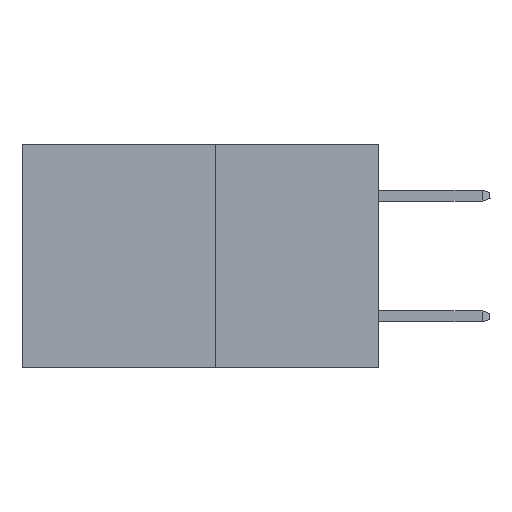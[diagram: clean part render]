
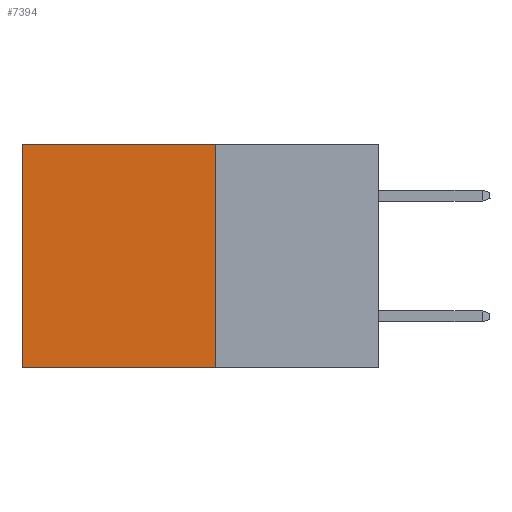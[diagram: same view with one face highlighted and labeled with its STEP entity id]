
A CAD part, left-side view. The second image highlights one B-rep face of the part: STEP entity #7394.
In plain terms, the highlighted planar face has unit normal (-1, 0, 0).
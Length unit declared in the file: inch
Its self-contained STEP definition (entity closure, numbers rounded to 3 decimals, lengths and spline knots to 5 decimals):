
#18 = DIRECTION ( 'NONE',  ( 0., 1., 0. ) ) ;
#302 = CARTESIAN_POINT ( 'NONE',  ( 0.277, 0.59, -0.37 ) ) ;
#645 = LINE ( 'NONE', #302, #13709 ) ;
#3429 = ORIENTED_EDGE ( 'NONE', *, *, #9623, .F. ) ;
#3603 = VECTOR ( 'NONE', #11856, 39.37008 ) ;
#4211 = CARTESIAN_POINT ( 'NONE',  ( 0.277, 0.27, -0.37 ) ) ;
#4755 = ORIENTED_EDGE ( 'NONE', *, *, #11557, .T. ) ;
#5382 = PLANE ( 'NONE',  #16140 ) ;
#5430 = DIRECTION ( 'NONE',  ( 0., 0., -1. ) ) ;
#5643 = LINE ( 'NONE', #14302, #9044 ) ;
#6697 = CARTESIAN_POINT ( 'NONE',  ( 0.277, 0.27, -0.37 ) ) ;
#6847 = LINE ( 'NONE', #6697, #3603 ) ;
#7394 = ADVANCED_FACE ( 'NONE', ( #8294 ), #5382, .F. ) ;
#7792 = DIRECTION ( 'NONE',  ( 0., 0., -1. ) ) ;
#8169 = EDGE_CURVE ( 'NONE', #11188, #9383, #6847, .T. ) ;
#8294 = FACE_OUTER_BOUND ( 'NONE', #8917, .T. ) ;
#8298 = ORIENTED_EDGE ( 'NONE', *, *, #8169, .F. ) ;
#8572 = CARTESIAN_POINT ( 'NONE',  ( 0.277, 0.59, 0. ) ) ;
#8891 = CARTESIAN_POINT ( 'NONE',  ( 0.277, 0.27, 0. ) ) ;
#8917 = EDGE_LOOP ( 'NONE', ( #4755, #3429, #8298, #10311 ) ) ;
#8935 = CARTESIAN_POINT ( 'NONE',  ( 0.277, 0.27, -0.37 ) ) ;
#9044 = VECTOR ( 'NONE', #10595, 39.37008 ) ;
#9276 = VECTOR ( 'NONE', #18, 39.37008 ) ;
#9383 = VERTEX_POINT ( 'NONE', #8935 ) ;
#9623 = EDGE_CURVE ( 'NONE', #9383, #9662, #5643, .T. ) ;
#9662 = VERTEX_POINT ( 'NONE', #14356 ) ;
#10311 = ORIENTED_EDGE ( 'NONE', *, *, #13713, .T. ) ;
#10595 = DIRECTION ( 'NONE',  ( 0., 1., 0. ) ) ;
#11188 = VERTEX_POINT ( 'NONE', #12228 ) ;
#11557 = EDGE_CURVE ( 'NONE', #14214, #9662, #645, .T. ) ;
#11856 = DIRECTION ( 'NONE',  ( 0., 0., -1. ) ) ;
#12228 = CARTESIAN_POINT ( 'NONE',  ( 0.277, 0.27, 0. ) ) ;
#12258 = LINE ( 'NONE', #8891, #9276 ) ;
#13037 = DIRECTION ( 'NONE',  ( 1., 0., 0. ) ) ;
#13709 = VECTOR ( 'NONE', #7792, 39.37008 ) ;
#13713 = EDGE_CURVE ( 'NONE', #11188, #14214, #12258, .T. ) ;
#14214 = VERTEX_POINT ( 'NONE', #8572 ) ;
#14302 = CARTESIAN_POINT ( 'NONE',  ( 0.277, 0.27, -0.37 ) ) ;
#14356 = CARTESIAN_POINT ( 'NONE',  ( 0.277, 0.59, -0.37 ) ) ;
#16140 = AXIS2_PLACEMENT_3D ( 'NONE', #4211, #13037, #5430 ) ;
